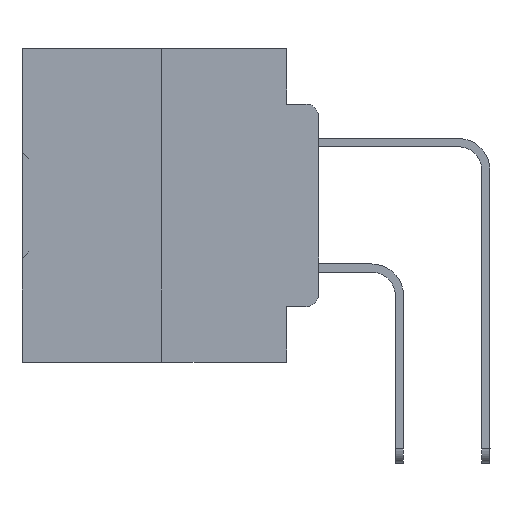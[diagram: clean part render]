
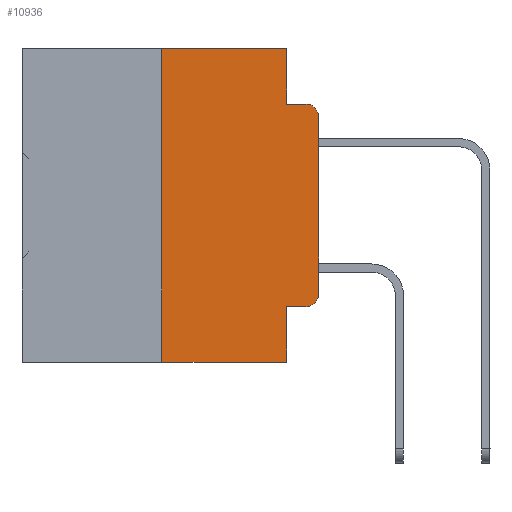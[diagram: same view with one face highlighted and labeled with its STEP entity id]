
A CAD part, left-side view. The second image highlights one B-rep face of the part: STEP entity #10936.
In plain terms, the highlighted planar face has unit normal (-1, 0, 0).
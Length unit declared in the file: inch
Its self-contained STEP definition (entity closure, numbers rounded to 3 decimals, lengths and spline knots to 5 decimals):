
#808 = EDGE_CURVE ( 'NONE', #31487, #31388, #30988, .T. ) ;
#1337 = VECTOR ( 'NONE', #24158, 39.37008 ) ;
#1534 = VECTOR ( 'NONE', #19055, 39.37008 ) ;
#1871 = EDGE_CURVE ( 'NONE', #30558, #24804, #5713, .T. ) ;
#2304 = DIRECTION ( 'NONE',  ( 0., -1., 0. ) ) ;
#2642 = LINE ( 'NONE', #15026, #37771 ) ;
#3827 = CARTESIAN_POINT ( 'NONE',  ( 0., 0.473, -0.5 ) ) ;
#4363 = ORIENTED_EDGE ( 'NONE', *, *, #1871, .F. ) ;
#4714 = CARTESIAN_POINT ( 'NONE',  ( 0., 0.02, -0.1085 ) ) ;
#5348 = CARTESIAN_POINT ( 'NONE',  ( 0., 0.473, 0. ) ) ;
#5372 = VERTEX_POINT ( 'NONE', #30890 ) ;
#5713 = LINE ( 'NONE', #18484, #1337 ) ;
#5782 = CARTESIAN_POINT ( 'NONE',  ( 0., 0.02, -0.4115 ) ) ;
#6974 = LINE ( 'NONE', #12470, #36827 ) ;
#7086 = AXIS2_PLACEMENT_3D ( 'NONE', #4714, #31611, #10985 ) ;
#7786 = VECTOR ( 'NONE', #15814, 39.37008 ) ;
#8374 = FACE_OUTER_BOUND ( 'NONE', #13295, .T. ) ;
#8683 = CARTESIAN_POINT ( 'NONE',  ( 0., 0., -0.3915 ) ) ;
#9521 = EDGE_CURVE ( 'NONE', #5372, #20821, #25502, .T. ) ;
#9888 = DIRECTION ( 'NONE',  ( 0., 0., -1. ) ) ;
#10275 = CARTESIAN_POINT ( 'NONE',  ( 0., 0.051, 0. ) ) ;
#10505 = EDGE_CURVE ( 'NONE', #11295, #37550, #6974, .T. ) ;
#10936 = ADVANCED_FACE ( 'NONE', ( #8374 ), #30018, .F. ) ;
#10985 = DIRECTION ( 'NONE',  ( 0., 0., -1. ) ) ;
#11295 = VERTEX_POINT ( 'NONE', #39303 ) ;
#11392 = VECTOR ( 'NONE', #2304, 39.37008 ) ;
#12470 = CARTESIAN_POINT ( 'NONE',  ( 0., 0.051, -0.4115 ) ) ;
#13295 = EDGE_LOOP ( 'NONE', ( #19898, #16033, #16119, #15162, #4363, #33340, #16078, #21536, #24060, #33512 ) ) ;
#14066 = DIRECTION ( 'NONE',  ( 0., 0., 1. ) ) ;
#14690 = DIRECTION ( 'NONE',  ( 0., 0., -1. ) ) ;
#14692 = CARTESIAN_POINT ( 'NONE',  ( 0., 0.051, -0.0885 ) ) ;
#15026 = CARTESIAN_POINT ( 'NONE',  ( 0., 0.051, 0. ) ) ;
#15162 = ORIENTED_EDGE ( 'NONE', *, *, #39980, .F. ) ;
#15814 = DIRECTION ( 'NONE',  ( 0., -1., 0. ) ) ;
#16033 = ORIENTED_EDGE ( 'NONE', *, *, #808, .T. ) ;
#16078 = ORIENTED_EDGE ( 'NONE', *, *, #9521, .T. ) ;
#16119 = ORIENTED_EDGE ( 'NONE', *, *, #34822, .F. ) ;
#16415 = CARTESIAN_POINT ( 'NONE',  ( 0., 0., 0. ) ) ;
#16496 = CARTESIAN_POINT ( 'NONE',  ( 0., 0.25, 0. ) ) ;
#16499 = CARTESIAN_POINT ( 'NONE',  ( 0., 0.02, -0.0885 ) ) ;
#16693 = CARTESIAN_POINT ( 'NONE',  ( 0., 0.02, -0.3915 ) ) ;
#17114 = DIRECTION ( 'NONE',  ( -1., 0., 0. ) ) ;
#17713 = DIRECTION ( 'NONE',  ( 1., 0., 0. ) ) ;
#17898 = EDGE_CURVE ( 'NONE', #11295, #20821, #25087, .T. ) ;
#18484 = CARTESIAN_POINT ( 'NONE',  ( 0., 0.473, 0. ) ) ;
#18699 = VECTOR ( 'NONE', #14066, 39.37008 ) ;
#18755 = CARTESIAN_POINT ( 'NONE',  ( 0., 0.051, -0.5 ) ) ;
#19055 = DIRECTION ( 'NONE',  ( 0., 0., 1. ) ) ;
#19127 = CARTESIAN_POINT ( 'NONE',  ( 0., 0.051, 0. ) ) ;
#19332 = DIRECTION ( 'NONE',  ( 0., -1., 0. ) ) ;
#19898 = ORIENTED_EDGE ( 'NONE', *, *, #21189, .T. ) ;
#20128 = CARTESIAN_POINT ( 'NONE',  ( 0., 0., -0.1085 ) ) ;
#20821 = VERTEX_POINT ( 'NONE', #18755 ) ;
#21189 = EDGE_CURVE ( 'NONE', #31193, #31487, #34787, .T. ) ;
#21280 = DIRECTION ( 'NONE',  ( 0., 0., -1. ) ) ;
#21536 = ORIENTED_EDGE ( 'NONE', *, *, #17898, .F. ) ;
#21652 = CARTESIAN_POINT ( 'NONE',  ( 0., 0.051, -0.0885 ) ) ;
#22570 = LINE ( 'NONE', #16496, #18699 ) ;
#24060 = ORIENTED_EDGE ( 'NONE', *, *, #10505, .T. ) ;
#24158 = DIRECTION ( 'NONE',  ( 0., -1., 0. ) ) ;
#24804 = VERTEX_POINT ( 'NONE', #19127 ) ;
#25087 = LINE ( 'NONE', #10275, #39562 ) ;
#25502 = LINE ( 'NONE', #3827, #7786 ) ;
#26825 = AXIS2_PLACEMENT_3D ( 'NONE', #16693, #17114, #32223 ) ;
#27612 = LINE ( 'NONE', #14692, #11392 ) ;
#27625 = EDGE_CURVE ( 'NONE', #5372, #30558, #22570, .T. ) ;
#27738 = AXIS2_PLACEMENT_3D ( 'NONE', #5348, #17713, #14690 ) ;
#30018 = PLANE ( 'NONE',  #27738 ) ;
#30558 = VERTEX_POINT ( 'NONE', #36550 ) ;
#30890 = CARTESIAN_POINT ( 'NONE',  ( 0., 0.25, -0.5 ) ) ;
#30988 = CIRCLE ( 'NONE', #7086, 0.02 ) ;
#31193 = VERTEX_POINT ( 'NONE', #8683 ) ;
#31388 = VERTEX_POINT ( 'NONE', #16499 ) ;
#31487 = VERTEX_POINT ( 'NONE', #20128 ) ;
#31611 = DIRECTION ( 'NONE',  ( -1., 0., 0. ) ) ;
#32223 = DIRECTION ( 'NONE',  ( 0., 0., -1. ) ) ;
#33340 = ORIENTED_EDGE ( 'NONE', *, *, #27625, .F. ) ;
#33385 = EDGE_CURVE ( 'NONE', #37550, #31193, #36482, .T. ) ;
#33512 = ORIENTED_EDGE ( 'NONE', *, *, #33385, .T. ) ;
#34013 = VERTEX_POINT ( 'NONE', #21652 ) ;
#34787 = LINE ( 'NONE', #16415, #1534 ) ;
#34822 = EDGE_CURVE ( 'NONE', #34013, #31388, #27612, .T. ) ;
#36482 = CIRCLE ( 'NONE', #26825, 0.02 ) ;
#36550 = CARTESIAN_POINT ( 'NONE',  ( 0., 0.25, 0. ) ) ;
#36827 = VECTOR ( 'NONE', #19332, 39.37008 ) ;
#37550 = VERTEX_POINT ( 'NONE', #5782 ) ;
#37771 = VECTOR ( 'NONE', #21280, 39.37008 ) ;
#39303 = CARTESIAN_POINT ( 'NONE',  ( 0., 0.051, -0.4115 ) ) ;
#39562 = VECTOR ( 'NONE', #9888, 39.37008 ) ;
#39980 = EDGE_CURVE ( 'NONE', #24804, #34013, #2642, .T. ) ;
